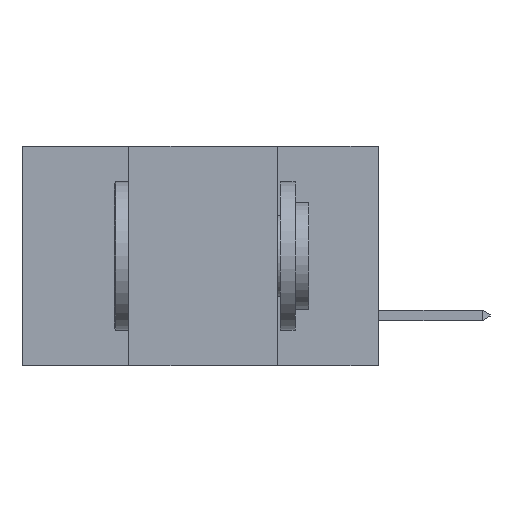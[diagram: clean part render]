
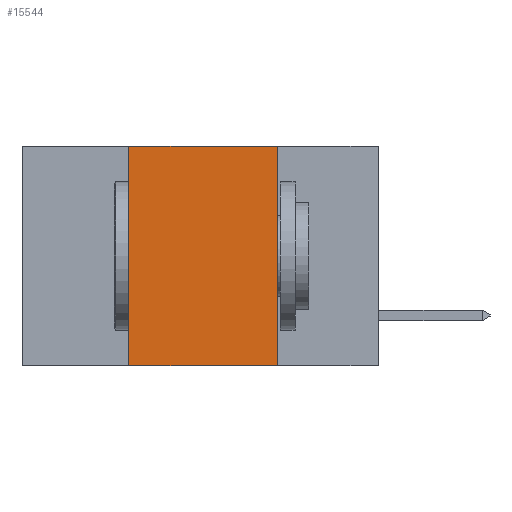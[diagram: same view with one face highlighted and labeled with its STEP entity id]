
A CAD part, left-side view. The second image highlights one B-rep face of the part: STEP entity #15544.
In plain terms, the highlighted planar face has unit normal (-1, 0, 0).
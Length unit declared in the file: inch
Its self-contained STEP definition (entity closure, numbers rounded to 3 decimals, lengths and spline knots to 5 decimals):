
#1545 = ORIENTED_EDGE ( 'NONE', *, *, #13887, .F. ) ;
#1793 = ORIENTED_EDGE ( 'NONE', *, *, #8843, .F. ) ;
#1987 = DIRECTION ( 'NONE',  ( 0., 0., 1. ) ) ;
#1991 = CARTESIAN_POINT ( 'NONE',  ( 0., 0.42, -0.37 ) ) ;
#2449 = EDGE_LOOP ( 'NONE', ( #1545, #1793, #3022, #3998 ) ) ;
#2791 = CARTESIAN_POINT ( 'NONE',  ( 0., 0.42, 0. ) ) ;
#3022 = ORIENTED_EDGE ( 'NONE', *, *, #7777, .F. ) ;
#3104 = VERTEX_POINT ( 'NONE', #2791 ) ;
#3911 = FACE_OUTER_BOUND ( 'NONE', #2449, .T. ) ;
#3998 = ORIENTED_EDGE ( 'NONE', *, *, #6745, .T. ) ;
#4861 = VECTOR ( 'NONE', #1987, 39.37008 ) ;
#6226 = DIRECTION ( 'NONE',  ( 0., 0., -1. ) ) ;
#6478 = CARTESIAN_POINT ( 'NONE',  ( 0., 0.17, -0.37 ) ) ;
#6745 = EDGE_CURVE ( 'NONE', #12072, #10328, #17100, .T. ) ;
#7626 = VECTOR ( 'NONE', #18773, 39.37008 ) ;
#7777 = EDGE_CURVE ( 'NONE', #12072, #3104, #8917, .T. ) ;
#7931 = DIRECTION ( 'NONE',  ( 0., 0., -1. ) ) ;
#8116 = LINE ( 'NONE', #18758, #7626 ) ;
#8843 = EDGE_CURVE ( 'NONE', #3104, #17005, #8116, .T. ) ;
#8917 = LINE ( 'NONE', #1991, #4861 ) ;
#9340 = CARTESIAN_POINT ( 'NONE',  ( 0., 0.6, -0.37 ) ) ;
#10328 = VERTEX_POINT ( 'NONE', #6478 ) ;
#10525 = DIRECTION ( 'NONE',  ( 0., -1., 0. ) ) ;
#10941 = CARTESIAN_POINT ( 'NONE',  ( 0., 0.6, 0. ) ) ;
#11069 = VECTOR ( 'NONE', #6226, 39.37008 ) ;
#11442 = CARTESIAN_POINT ( 'NONE',  ( 0., 0.42, -0.37 ) ) ;
#12072 = VERTEX_POINT ( 'NONE', #11442 ) ;
#13085 = AXIS2_PLACEMENT_3D ( 'NONE', #10941, #16890, #7931 ) ;
#13240 = VECTOR ( 'NONE', #10525, 39.37008 ) ;
#13887 = EDGE_CURVE ( 'NONE', #17005, #10328, #15041, .T. ) ;
#13968 = PLANE ( 'NONE',  #13085 ) ;
#15041 = LINE ( 'NONE', #16806, #11069 ) ;
#15544 = ADVANCED_FACE ( 'NONE', ( #3911 ), #13968, .F. ) ;
#15714 = CARTESIAN_POINT ( 'NONE',  ( 0., 0.17, 0. ) ) ;
#16806 = CARTESIAN_POINT ( 'NONE',  ( 0., 0.17, -0.37 ) ) ;
#16890 = DIRECTION ( 'NONE',  ( 1., 0., 0. ) ) ;
#17005 = VERTEX_POINT ( 'NONE', #15714 ) ;
#17100 = LINE ( 'NONE', #9340, #13240 ) ;
#18758 = CARTESIAN_POINT ( 'NONE',  ( 0., 0.6, 0. ) ) ;
#18773 = DIRECTION ( 'NONE',  ( 0., -1., 0. ) ) ;
